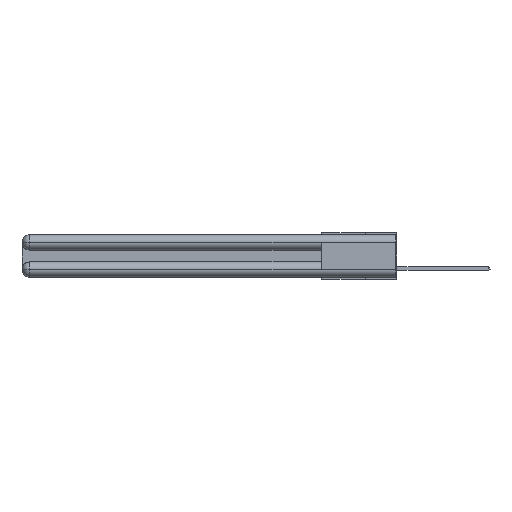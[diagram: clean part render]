
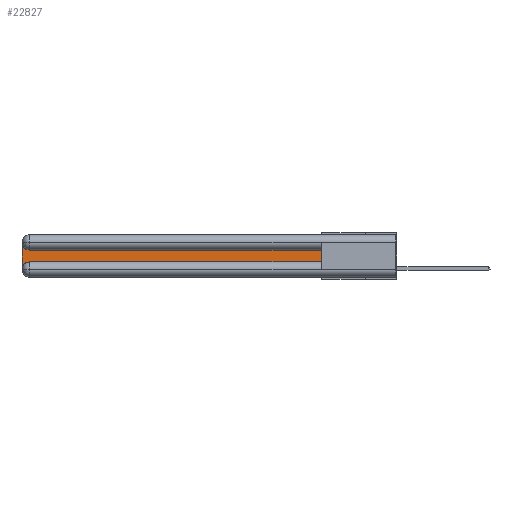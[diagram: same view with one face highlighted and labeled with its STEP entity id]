
A CAD part, left-side view. The second image highlights one B-rep face of the part: STEP entity #22827.
In plain terms, the highlighted planar face has unit normal (-1, 0, 0).
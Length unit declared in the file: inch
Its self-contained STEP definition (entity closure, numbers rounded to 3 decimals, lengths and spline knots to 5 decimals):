
#210 = CARTESIAN_POINT ( 'NONE',  ( 0.075, 0.6, -0.1225 ) ) ;
#986 = CIRCLE ( 'NONE', #32859, 0.06 ) ;
#2150 = LINE ( 'NONE', #30299, #22204 ) ;
#2515 = DIRECTION ( 'NONE',  ( 0., 0., 1. ) ) ;
#2764 = DIRECTION ( 'NONE',  ( 1., 0., 0. ) ) ;
#2994 = CARTESIAN_POINT ( 'NONE',  ( 0.075, 3., -0.1225 ) ) ;
#5532 = DIRECTION ( 'NONE',  ( 0., 0., -1. ) ) ;
#5899 = CIRCLE ( 'NONE', #16831, 0.06 ) ;
#6330 = EDGE_CURVE ( 'NONE', #30117, #26024, #5899, .T. ) ;
#8547 = VERTEX_POINT ( 'NONE', #9167 ) ;
#9167 = CARTESIAN_POINT ( 'NONE',  ( 0.075, 3., -0.0625 ) ) ;
#9372 = ORIENTED_EDGE ( 'NONE', *, *, #12783, .T. ) ;
#11264 = VERTEX_POINT ( 'NONE', #32227 ) ;
#12783 = EDGE_CURVE ( 'NONE', #11264, #24352, #23036, .T. ) ;
#13989 = ORIENTED_EDGE ( 'NONE', *, *, #18841, .T. ) ;
#14862 = VECTOR ( 'NONE', #2515, 39.37008 ) ;
#16008 = CARTESIAN_POINT ( 'NONE',  ( 0.075, 2.94, -0.2775 ) ) ;
#16831 = AXIS2_PLACEMENT_3D ( 'NONE', #16008, #2764, #18423 ) ;
#18423 = DIRECTION ( 'NONE',  ( 0., 0., -1. ) ) ;
#18485 = VERTEX_POINT ( 'NONE', #32873 ) ;
#18841 = EDGE_CURVE ( 'NONE', #24352, #18485, #25269, .T. ) ;
#19408 = ORIENTED_EDGE ( 'NONE', *, *, #6330, .T. ) ;
#19498 = CARTESIAN_POINT ( 'NONE',  ( 0.075, 2.94, -0.2175 ) ) ;
#20961 = PLANE ( 'NONE',  #22719 ) ;
#22204 = VECTOR ( 'NONE', #27327, 39.37008 ) ;
#22378 = ORIENTED_EDGE ( 'NONE', *, *, #26491, .T. ) ;
#22719 = AXIS2_PLACEMENT_3D ( 'NONE', #2994, #31531, #5532 ) ;
#22827 = ADVANCED_FACE ( 'NONE', ( #28109 ), #20961, .F. ) ;
#23036 = LINE ( 'NONE', #28945, #14862 ) ;
#24221 = ORIENTED_EDGE ( 'NONE', *, *, #25894, .T. ) ;
#24352 = VERTEX_POINT ( 'NONE', #210 ) ;
#24867 = CARTESIAN_POINT ( 'NONE',  ( 0.075, 3., -0.2775 ) ) ;
#25269 = LINE ( 'NONE', #29301, #30178 ) ;
#25618 = EDGE_LOOP ( 'NONE', ( #13989, #32983, #24221, #19408, #22378, #9372 ) ) ;
#25840 = LINE ( 'NONE', #26247, #26238 ) ;
#25891 = DIRECTION ( 'NONE',  ( 1., 0., 0. ) ) ;
#25894 = EDGE_CURVE ( 'NONE', #8547, #30117, #2150, .T. ) ;
#26024 = VERTEX_POINT ( 'NONE', #19498 ) ;
#26238 = VECTOR ( 'NONE', #31205, 39.37008 ) ;
#26247 = CARTESIAN_POINT ( 'NONE',  ( 0.075, 0.6, -0.2175 ) ) ;
#26491 = EDGE_CURVE ( 'NONE', #26024, #11264, #25840, .T. ) ;
#27327 = DIRECTION ( 'NONE',  ( 0., 0., -1. ) ) ;
#28109 = FACE_OUTER_BOUND ( 'NONE', #25618, .T. ) ;
#28945 = CARTESIAN_POINT ( 'NONE',  ( 0.075, 0.6, -0.2175 ) ) ;
#29301 = CARTESIAN_POINT ( 'NONE',  ( 0.075, 0.6, -0.1225 ) ) ;
#29550 = DIRECTION ( 'NONE',  ( 0., 1., 0. ) ) ;
#30117 = VERTEX_POINT ( 'NONE', #24867 ) ;
#30178 = VECTOR ( 'NONE', #29550, 39.37008 ) ;
#30299 = CARTESIAN_POINT ( 'NONE',  ( 0.075, 3., -0.2175 ) ) ;
#30967 = CARTESIAN_POINT ( 'NONE',  ( 0.075, 2.94, -0.0625 ) ) ;
#31205 = DIRECTION ( 'NONE',  ( 0., -1., 0. ) ) ;
#31316 = DIRECTION ( 'NONE',  ( 0., 0., -1. ) ) ;
#31386 = EDGE_CURVE ( 'NONE', #18485, #8547, #986, .T. ) ;
#31531 = DIRECTION ( 'NONE',  ( 1., 0., 0. ) ) ;
#32227 = CARTESIAN_POINT ( 'NONE',  ( 0.075, 0.6, -0.2175 ) ) ;
#32859 = AXIS2_PLACEMENT_3D ( 'NONE', #30967, #25891, #31316 ) ;
#32873 = CARTESIAN_POINT ( 'NONE',  ( 0.075, 2.94, -0.1225 ) ) ;
#32983 = ORIENTED_EDGE ( 'NONE', *, *, #31386, .T. ) ;
